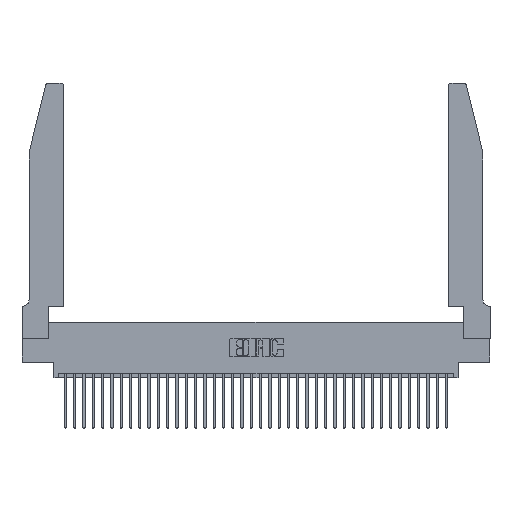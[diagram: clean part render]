
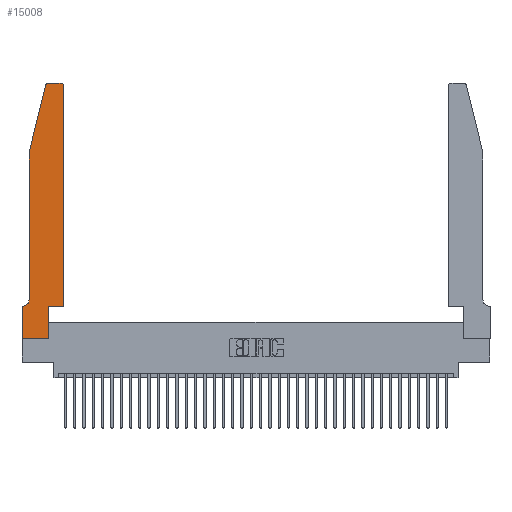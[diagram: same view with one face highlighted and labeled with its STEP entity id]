
A CAD part, top view. The second image highlights one B-rep face of the part: STEP entity #15008.
In plain terms, the highlighted planar face has unit normal (0, 0, 1).
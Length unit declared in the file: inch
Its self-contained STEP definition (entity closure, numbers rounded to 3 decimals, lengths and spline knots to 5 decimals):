
#349 = CIRCLE ( 'NONE', #12870, 0.03 ) ;
#372 = CARTESIAN_POINT ( 'NONE',  ( 0.2865, 0., 0.37 ) ) ;
#707 = DIRECTION ( 'NONE',  ( -0.239, -0.971, 0. ) ) ;
#1917 = ORIENTED_EDGE ( 'NONE', *, *, #19336, .T. ) ;
#2047 = LINE ( 'NONE', #28738, #16932 ) ;
#2140 = DIRECTION ( 'NONE',  ( 0., 1., 0. ) ) ;
#3225 = DIRECTION ( 'NONE',  ( 0., 0., -1. ) ) ;
#3296 = EDGE_CURVE ( 'NONE', #32472, #22026, #22395, .T. ) ;
#3373 = LINE ( 'NONE', #12708, #17312 ) ;
#3519 = CARTESIAN_POINT ( 'NONE',  ( 0.4205, 2.72, 0.37 ) ) ;
#3924 = LINE ( 'NONE', #25699, #18727 ) ;
#4055 = CARTESIAN_POINT ( 'NONE',  ( 0.0055, 0.35, 0.37 ) ) ;
#4405 = CIRCLE ( 'NONE', #11340, 0.07 ) ;
#4769 = CARTESIAN_POINT ( 'NONE',  ( 0.284, 2.72, 0.37 ) ) ;
#5167 = CARTESIAN_POINT ( 'NONE',  ( 0., 0.35, 0.37 ) ) ;
#6519 = DIRECTION ( 'NONE',  ( 1., 0., 0. ) ) ;
#6622 = ORIENTED_EDGE ( 'NONE', *, *, #27751, .T. ) ;
#6951 = CARTESIAN_POINT ( 'NONE',  ( 0.4505, 2.72, 0.37 ) ) ;
#7069 = CARTESIAN_POINT ( 'NONE',  ( 0.4505, 0.35, 0.37 ) ) ;
#7305 = EDGE_CURVE ( 'NONE', #24341, #36105, #3924, .T. ) ;
#7360 = EDGE_CURVE ( 'NONE', #11501, #26593, #2047, .T. ) ;
#7511 = AXIS2_PLACEMENT_3D ( 'NONE', #3519, #24113, #6519 ) ;
#7749 = DIRECTION ( 'NONE',  ( 1., 0., 0. ) ) ;
#7774 = CARTESIAN_POINT ( 'NONE',  ( 0.0755, 0.35, 0.37 ) ) ;
#7985 = CARTESIAN_POINT ( 'NONE',  ( 0.4505, 0.35, 0.37 ) ) ;
#7990 = ORIENTED_EDGE ( 'NONE', *, *, #3296, .T. ) ;
#8149 = DIRECTION ( 'NONE',  ( 1., 0., 0. ) ) ;
#8794 = FACE_OUTER_BOUND ( 'NONE', #22281, .T. ) ;
#9238 = VERTEX_POINT ( 'NONE', #4055 ) ;
#9466 = LINE ( 'NONE', #27949, #18235 ) ;
#10066 = DIRECTION ( 'NONE',  ( 0., 1., 0. ) ) ;
#10449 = DIRECTION ( 'NONE',  ( 1., 0., 0. ) ) ;
#10874 = DIRECTION ( 'NONE',  ( 0., -1., 0. ) ) ;
#11329 = CARTESIAN_POINT ( 'NONE',  ( 0., 0.35, 0.37 ) ) ;
#11340 = AXIS2_PLACEMENT_3D ( 'NONE', #20926, #3225, #23832 ) ;
#11501 = VERTEX_POINT ( 'NONE', #11329 ) ;
#11614 = VERTEX_POINT ( 'NONE', #35200 ) ;
#12708 = CARTESIAN_POINT ( 'NONE',  ( 0.0755, 2., 0.37 ) ) ;
#12870 = AXIS2_PLACEMENT_3D ( 'NONE', #4769, #25307, #7749 ) ;
#13162 = CARTESIAN_POINT ( 'NONE',  ( 0.2605, 2.75, 0.37 ) ) ;
#13228 = EDGE_CURVE ( 'NONE', #26593, #24341, #26979, .T. ) ;
#13975 = CARTESIAN_POINT ( 'NONE',  ( 0.2865, 0.35, 0.37 ) ) ;
#14500 = CARTESIAN_POINT ( 'NONE',  ( 0.25487, 2.72718, 0.37 ) ) ;
#14650 = VECTOR ( 'NONE', #21965, 39.37008 ) ;
#15008 = ADVANCED_FACE ( 'NONE', ( #8794 ), #37113, .T. ) ;
#15852 = ORIENTED_EDGE ( 'NONE', *, *, #18199, .T. ) ;
#15873 = ORIENTED_EDGE ( 'NONE', *, *, #36034, .T. ) ;
#16245 = VERTEX_POINT ( 'NONE', #34043 ) ;
#16279 = LINE ( 'NONE', #7069, #23090 ) ;
#16932 = VECTOR ( 'NONE', #17212, 39.37008 ) ;
#17212 = DIRECTION ( 'NONE',  ( 0., -1., 0. ) ) ;
#17312 = VECTOR ( 'NONE', #707, 39.37008 ) ;
#18194 = CIRCLE ( 'NONE', #7511, 0.03 ) ;
#18199 = EDGE_CURVE ( 'NONE', #36105, #26552, #9466, .T. ) ;
#18235 = VECTOR ( 'NONE', #10449, 39.37008 ) ;
#18610 = EDGE_CURVE ( 'NONE', #28142, #32472, #18194, .T. ) ;
#18727 = VECTOR ( 'NONE', #2140, 39.37008 ) ;
#19038 = CARTESIAN_POINT ( 'NONE',  ( 0.284, 2.75, 0.37 ) ) ;
#19314 = VECTOR ( 'NONE', #25326, 39.37008 ) ;
#19336 = EDGE_CURVE ( 'NONE', #25507, #11614, #3373, .T. ) ;
#19955 = CARTESIAN_POINT ( 'NONE',  ( 0., 0., 0.37 ) ) ;
#20926 = CARTESIAN_POINT ( 'NONE',  ( 0.0055, 0.42, 0.37 ) ) ;
#21301 = VECTOR ( 'NONE', #10874, 39.37008 ) ;
#21484 = AXIS2_PLACEMENT_3D ( 'NONE', #5167, #25700, #8149 ) ;
#21965 = DIRECTION ( 'NONE',  ( -1., 0., 0. ) ) ;
#22026 = VERTEX_POINT ( 'NONE', #19038 ) ;
#22281 = EDGE_LOOP ( 'NONE', ( #7990, #15873, #1917, #6622, #36681, #31291, #23605, #36222, #25401, #15852, #22905, #34448 ) ) ;
#22395 = LINE ( 'NONE', #13162, #14650 ) ;
#22506 = EDGE_CURVE ( 'NONE', #16245, #9238, #4405, .T. ) ;
#22527 = CARTESIAN_POINT ( 'NONE',  ( 0.0755, 2., 0.37 ) ) ;
#22905 = ORIENTED_EDGE ( 'NONE', *, *, #28115, .T. ) ;
#23090 = VECTOR ( 'NONE', #10066, 39.37008 ) ;
#23605 = ORIENTED_EDGE ( 'NONE', *, *, #7360, .T. ) ;
#23832 = DIRECTION ( 'NONE',  ( -1., 0., 0. ) ) ;
#24113 = DIRECTION ( 'NONE',  ( 0., 0., 1. ) ) ;
#24341 = VERTEX_POINT ( 'NONE', #372 ) ;
#25307 = DIRECTION ( 'NONE',  ( 0., 0., 1. ) ) ;
#25326 = DIRECTION ( 'NONE',  ( -1., 0., 0. ) ) ;
#25401 = ORIENTED_EDGE ( 'NONE', *, *, #7305, .T. ) ;
#25507 = VERTEX_POINT ( 'NONE', #14500 ) ;
#25699 = CARTESIAN_POINT ( 'NONE',  ( 0.2865, 0.35, 0.37 ) ) ;
#25700 = DIRECTION ( 'NONE',  ( 0., 0., 1. ) ) ;
#26552 = VERTEX_POINT ( 'NONE', #7985 ) ;
#26593 = VERTEX_POINT ( 'NONE', #19955 ) ;
#26979 = LINE ( 'NONE', #28442, #32805 ) ;
#27045 = LINE ( 'NONE', #7774, #19314 ) ;
#27751 = EDGE_CURVE ( 'NONE', #11614, #16245, #30808, .T. ) ;
#27949 = CARTESIAN_POINT ( 'NONE',  ( 0.4505, 0.35, 0.37 ) ) ;
#28115 = EDGE_CURVE ( 'NONE', #26552, #28142, #16279, .T. ) ;
#28142 = VERTEX_POINT ( 'NONE', #6951 ) ;
#28274 = CARTESIAN_POINT ( 'NONE',  ( 0.4205, 2.75, 0.37 ) ) ;
#28442 = CARTESIAN_POINT ( 'NONE',  ( 0., 0., 0.37 ) ) ;
#28738 = CARTESIAN_POINT ( 'NONE',  ( 0., 0., 0.37 ) ) ;
#30748 = EDGE_CURVE ( 'NONE', #9238, #11501, #27045, .T. ) ;
#30808 = LINE ( 'NONE', #22527, #21301 ) ;
#31291 = ORIENTED_EDGE ( 'NONE', *, *, #30748, .T. ) ;
#32472 = VERTEX_POINT ( 'NONE', #28274 ) ;
#32805 = VECTOR ( 'NONE', #34197, 39.37008 ) ;
#34043 = CARTESIAN_POINT ( 'NONE',  ( 0.0755, 0.42, 0.37 ) ) ;
#34197 = DIRECTION ( 'NONE',  ( 1., 0., 0. ) ) ;
#34448 = ORIENTED_EDGE ( 'NONE', *, *, #18610, .T. ) ;
#35200 = CARTESIAN_POINT ( 'NONE',  ( 0.0755, 2., 0.37 ) ) ;
#36034 = EDGE_CURVE ( 'NONE', #22026, #25507, #349, .T. ) ;
#36105 = VERTEX_POINT ( 'NONE', #13975 ) ;
#36222 = ORIENTED_EDGE ( 'NONE', *, *, #13228, .T. ) ;
#36681 = ORIENTED_EDGE ( 'NONE', *, *, #22506, .T. ) ;
#37113 = PLANE ( 'NONE',  #21484 ) ;
